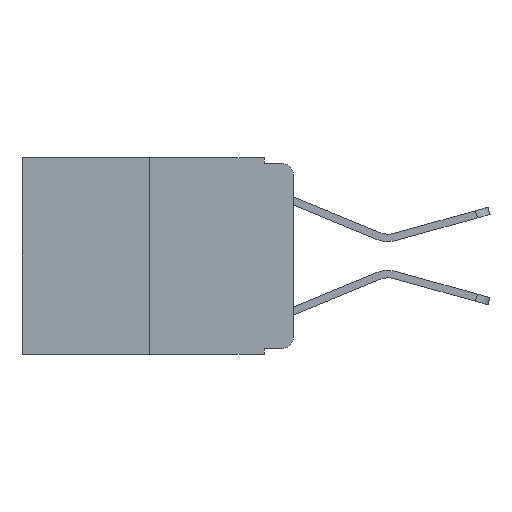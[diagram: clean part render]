
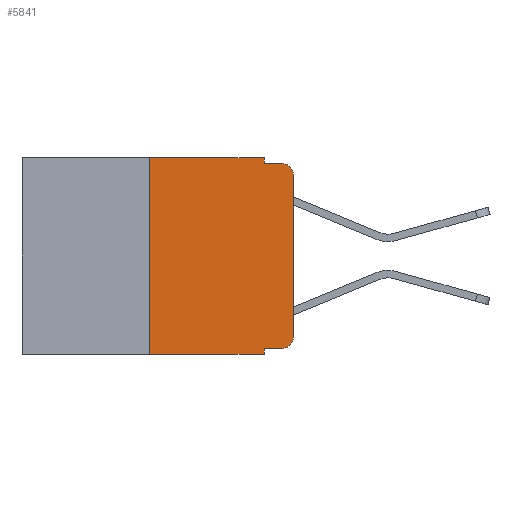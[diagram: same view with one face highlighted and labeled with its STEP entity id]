
A CAD part, left-side view. The second image highlights one B-rep face of the part: STEP entity #5841.
In plain terms, the highlighted planar face has unit normal (-1, 0, 0).
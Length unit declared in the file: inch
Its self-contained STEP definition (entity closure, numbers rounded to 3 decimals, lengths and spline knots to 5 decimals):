
#153 = CARTESIAN_POINT ( 'NONE',  ( 0., 0.25, 0. ) ) ;
#171 = CARTESIAN_POINT ( 'NONE',  ( 0., 0., -0.313 ) ) ;
#241 = LINE ( 'NONE', #4797, #2646 ) ;
#414 = CIRCLE ( 'NONE', #5952, 0.02 ) ;
#511 = VECTOR ( 'NONE', #8205, 39.37008 ) ;
#531 = DIRECTION ( 'NONE',  ( 1., 0., 0. ) ) ;
#559 = DIRECTION ( 'NONE',  ( 0., 0., -1. ) ) ;
#589 = FACE_OUTER_BOUND ( 'NONE', #6452, .T. ) ;
#665 = LINE ( 'NONE', #6750, #3161 ) ;
#810 = LINE ( 'NONE', #8674, #3261 ) ;
#866 = VERTEX_POINT ( 'NONE', #1209 ) ;
#885 = ORIENTED_EDGE ( 'NONE', *, *, #8123, .T. ) ;
#939 = CARTESIAN_POINT ( 'NONE',  ( 0., 0.02, -0.01 ) ) ;
#1010 = CARTESIAN_POINT ( 'NONE',  ( 0., 0.02, -0.313 ) ) ;
#1209 = CARTESIAN_POINT ( 'NONE',  ( 0., 0.25, 0. ) ) ;
#1219 = VECTOR ( 'NONE', #8956, 39.37008 ) ;
#1276 = LINE ( 'NONE', #7154, #6001 ) ;
#1329 = DIRECTION ( 'NONE',  ( 0., 0., -1. ) ) ;
#1352 = CARTESIAN_POINT ( 'NONE',  ( 0., 0.473, 0. ) ) ;
#1690 = CARTESIAN_POINT ( 'NONE',  ( 0., 0.02, -0.333 ) ) ;
#1798 = EDGE_CURVE ( 'NONE', #6554, #5705, #8993, .T. ) ;
#1951 = EDGE_CURVE ( 'NONE', #4102, #2160, #8269, .T. ) ;
#2137 = LINE ( 'NONE', #1352, #1219 ) ;
#2160 = VERTEX_POINT ( 'NONE', #939 ) ;
#2393 = CARTESIAN_POINT ( 'NONE',  ( 0., 0.051, -0.01 ) ) ;
#2625 = CARTESIAN_POINT ( 'NONE',  ( 0., 0.25, -0.343 ) ) ;
#2646 = VECTOR ( 'NONE', #3962, 39.37008 ) ;
#2685 = EDGE_CURVE ( 'NONE', #8339, #866, #7120, .T. ) ;
#2868 = DIRECTION ( 'NONE',  ( 0., 0., 1. ) ) ;
#2888 = EDGE_CURVE ( 'NONE', #866, #7401, #2137, .T. ) ;
#3078 = AXIS2_PLACEMENT_3D ( 'NONE', #4657, #531, #3824 ) ;
#3092 = VECTOR ( 'NONE', #1329, 39.37008 ) ;
#3161 = VECTOR ( 'NONE', #4904, 39.37008 ) ;
#3224 = VERTEX_POINT ( 'NONE', #10334 ) ;
#3261 = VECTOR ( 'NONE', #10221, 39.37008 ) ;
#3528 = CARTESIAN_POINT ( 'NONE',  ( 0., 0.051, -0.333 ) ) ;
#3824 = DIRECTION ( 'NONE',  ( 0., 0., -1. ) ) ;
#3864 = ORIENTED_EDGE ( 'NONE', *, *, #1951, .F. ) ;
#3962 = DIRECTION ( 'NONE',  ( 0., 0., 1. ) ) ;
#4021 = LINE ( 'NONE', #6475, #3092 ) ;
#4102 = VERTEX_POINT ( 'NONE', #6216 ) ;
#4409 = EDGE_CURVE ( 'NONE', #5009, #6554, #810, .T. ) ;
#4657 = CARTESIAN_POINT ( 'NONE',  ( 0., 0.473, 0. ) ) ;
#4797 = CARTESIAN_POINT ( 'NONE',  ( 0., 0., 0. ) ) ;
#4904 = DIRECTION ( 'NONE',  ( 0., 0., -1. ) ) ;
#5009 = VERTEX_POINT ( 'NONE', #3528 ) ;
#5071 = EDGE_CURVE ( 'NONE', #5009, #6792, #4021, .T. ) ;
#5336 = VECTOR ( 'NONE', #2868, 39.37008 ) ;
#5418 = CARTESIAN_POINT ( 'NONE',  ( 0., 0.051, -0.343 ) ) ;
#5488 = ORIENTED_EDGE ( 'NONE', *, *, #4409, .T. ) ;
#5645 = CARTESIAN_POINT ( 'NONE',  ( 0., 0.02, -0.03 ) ) ;
#5705 = VERTEX_POINT ( 'NONE', #171 ) ;
#5841 = ADVANCED_FACE ( 'NONE', ( #589 ), #6561, .F. ) ;
#5952 = AXIS2_PLACEMENT_3D ( 'NONE', #5645, #8213, #559 ) ;
#6001 = VECTOR ( 'NONE', #9973, 39.37008 ) ;
#6216 = CARTESIAN_POINT ( 'NONE',  ( 0., 0.051, -0.01 ) ) ;
#6452 = EDGE_LOOP ( 'NONE', ( #10368, #6920, #3864, #6583, #8358, #7983, #885, #10616, #5488, #8188 ) ) ;
#6475 = CARTESIAN_POINT ( 'NONE',  ( 0., 0.051, 0. ) ) ;
#6554 = VERTEX_POINT ( 'NONE', #1690 ) ;
#6561 = PLANE ( 'NONE',  #3078 ) ;
#6583 = ORIENTED_EDGE ( 'NONE', *, *, #8630, .F. ) ;
#6638 = CARTESIAN_POINT ( 'NONE',  ( 0., 0.051, 0. ) ) ;
#6687 = AXIS2_PLACEMENT_3D ( 'NONE', #1010, #6944, #7833 ) ;
#6750 = CARTESIAN_POINT ( 'NONE',  ( 0., 0.051, 0. ) ) ;
#6792 = VERTEX_POINT ( 'NONE', #5418 ) ;
#6888 = EDGE_CURVE ( 'NONE', #3224, #2160, #414, .T. ) ;
#6920 = ORIENTED_EDGE ( 'NONE', *, *, #6888, .T. ) ;
#6944 = DIRECTION ( 'NONE',  ( -1., 0., 0. ) ) ;
#7120 = LINE ( 'NONE', #153, #5336 ) ;
#7154 = CARTESIAN_POINT ( 'NONE',  ( 0., 0.473, -0.343 ) ) ;
#7401 = VERTEX_POINT ( 'NONE', #6638 ) ;
#7833 = DIRECTION ( 'NONE',  ( 0., 0., -1. ) ) ;
#7983 = ORIENTED_EDGE ( 'NONE', *, *, #2685, .F. ) ;
#8123 = EDGE_CURVE ( 'NONE', #8339, #6792, #1276, .T. ) ;
#8188 = ORIENTED_EDGE ( 'NONE', *, *, #1798, .T. ) ;
#8205 = DIRECTION ( 'NONE',  ( 0., -1., 0. ) ) ;
#8213 = DIRECTION ( 'NONE',  ( -1., 0., 0. ) ) ;
#8269 = LINE ( 'NONE', #2393, #511 ) ;
#8339 = VERTEX_POINT ( 'NONE', #2625 ) ;
#8358 = ORIENTED_EDGE ( 'NONE', *, *, #2888, .F. ) ;
#8630 = EDGE_CURVE ( 'NONE', #7401, #4102, #665, .T. ) ;
#8674 = CARTESIAN_POINT ( 'NONE',  ( 0., 0.051, -0.333 ) ) ;
#8956 = DIRECTION ( 'NONE',  ( 0., -1., 0. ) ) ;
#8993 = CIRCLE ( 'NONE', #6687, 0.02 ) ;
#9788 = EDGE_CURVE ( 'NONE', #5705, #3224, #241, .T. ) ;
#9973 = DIRECTION ( 'NONE',  ( 0., -1., 0. ) ) ;
#10221 = DIRECTION ( 'NONE',  ( 0., -1., 0. ) ) ;
#10334 = CARTESIAN_POINT ( 'NONE',  ( 0., 0., -0.03 ) ) ;
#10368 = ORIENTED_EDGE ( 'NONE', *, *, #9788, .T. ) ;
#10616 = ORIENTED_EDGE ( 'NONE', *, *, #5071, .F. ) ;
